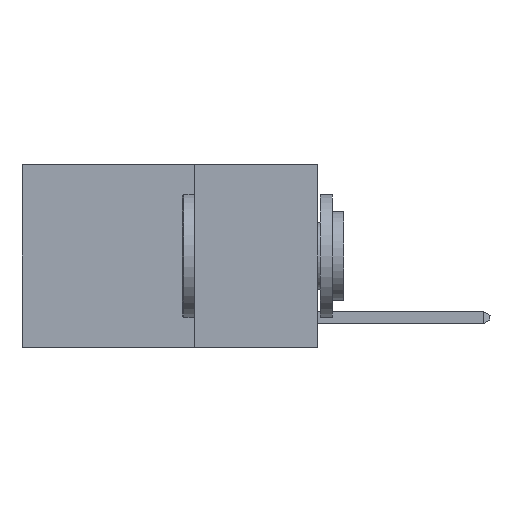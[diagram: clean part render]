
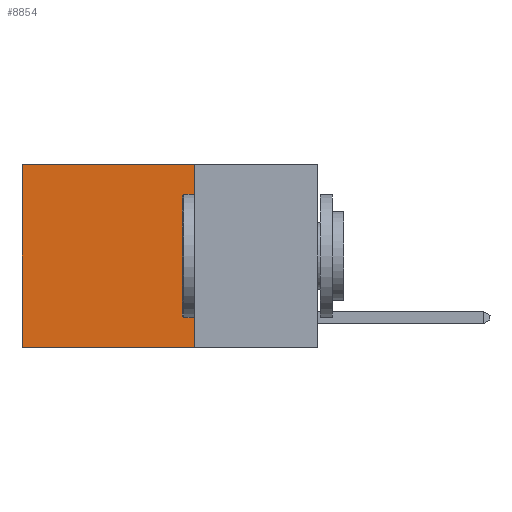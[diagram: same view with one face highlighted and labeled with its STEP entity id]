
A CAD part, left-side view. The second image highlights one B-rep face of the part: STEP entity #8854.
In plain terms, the highlighted planar face has unit normal (-1, 0, 0).
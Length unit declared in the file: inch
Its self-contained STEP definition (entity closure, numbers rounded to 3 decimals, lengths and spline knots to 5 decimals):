
#172 = VECTOR ( 'NONE', #2570, 39.37008 ) ;
#324 = ORIENTED_EDGE ( 'NONE', *, *, #2459, .T. ) ;
#1216 = EDGE_CURVE ( 'NONE', #4736, #6038, #13531, .T. ) ;
#1440 = AXIS2_PLACEMENT_3D ( 'NONE', #10774, #6591, #8779 ) ;
#1834 = DIRECTION ( 'NONE',  ( 0., 0., -1. ) ) ;
#2228 = VERTEX_POINT ( 'NONE', #10198 ) ;
#2459 = EDGE_CURVE ( 'NONE', #4736, #2228, #11386, .T. ) ;
#2570 = DIRECTION ( 'NONE',  ( 0., 0., -1. ) ) ;
#2888 = DIRECTION ( 'NONE',  ( 0., 1., 0. ) ) ;
#4736 = VERTEX_POINT ( 'NONE', #6880 ) ;
#5348 = ORIENTED_EDGE ( 'NONE', *, *, #8186, .T. ) ;
#5680 = CARTESIAN_POINT ( 'NONE',  ( 0.2625, 0.25, 0. ) ) ;
#5810 = CARTESIAN_POINT ( 'NONE',  ( 0.2625, 0.25, -0.37 ) ) ;
#5815 = LINE ( 'NONE', #7999, #7331 ) ;
#5867 = DIRECTION ( 'NONE',  ( 0., 1., 0. ) ) ;
#6038 = VERTEX_POINT ( 'NONE', #5810 ) ;
#6178 = ORIENTED_EDGE ( 'NONE', *, *, #1216, .F. ) ;
#6591 = DIRECTION ( 'NONE',  ( 1., 0., 0. ) ) ;
#6880 = CARTESIAN_POINT ( 'NONE',  ( 0.2625, 0.25, 0. ) ) ;
#7087 = VERTEX_POINT ( 'NONE', #10014 ) ;
#7331 = VECTOR ( 'NONE', #1834, 39.37008 ) ;
#7789 = PLANE ( 'NONE',  #1440 ) ;
#7999 = CARTESIAN_POINT ( 'NONE',  ( 0.2625, 0.6, 0. ) ) ;
#8186 = EDGE_CURVE ( 'NONE', #2228, #7087, #5815, .T. ) ;
#8779 = DIRECTION ( 'NONE',  ( 0., 0., -1. ) ) ;
#8854 = ADVANCED_FACE ( 'NONE', ( #9698 ), #7789, .F. ) ;
#9165 = CARTESIAN_POINT ( 'NONE',  ( 0.2625, 0.25, 0. ) ) ;
#9698 = FACE_OUTER_BOUND ( 'NONE', #12874, .T. ) ;
#10014 = CARTESIAN_POINT ( 'NONE',  ( 0.2625, 0.6, -0.37 ) ) ;
#10198 = CARTESIAN_POINT ( 'NONE',  ( 0.2625, 0.6, 0. ) ) ;
#10774 = CARTESIAN_POINT ( 'NONE',  ( 0.2625, 0.25, 0. ) ) ;
#11012 = VECTOR ( 'NONE', #2888, 39.37008 ) ;
#11292 = ORIENTED_EDGE ( 'NONE', *, *, #11613, .F. ) ;
#11381 = CARTESIAN_POINT ( 'NONE',  ( 0.2625, 0.25, -0.37 ) ) ;
#11386 = LINE ( 'NONE', #9165, #11012 ) ;
#11613 = EDGE_CURVE ( 'NONE', #6038, #7087, #13433, .T. ) ;
#12874 = EDGE_LOOP ( 'NONE', ( #5348, #11292, #6178, #324 ) ) ;
#13433 = LINE ( 'NONE', #11381, #13594 ) ;
#13531 = LINE ( 'NONE', #5680, #172 ) ;
#13594 = VECTOR ( 'NONE', #5867, 39.37008 ) ;
